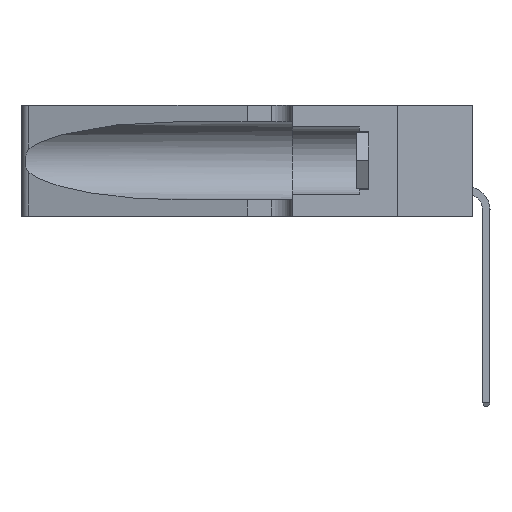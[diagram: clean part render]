
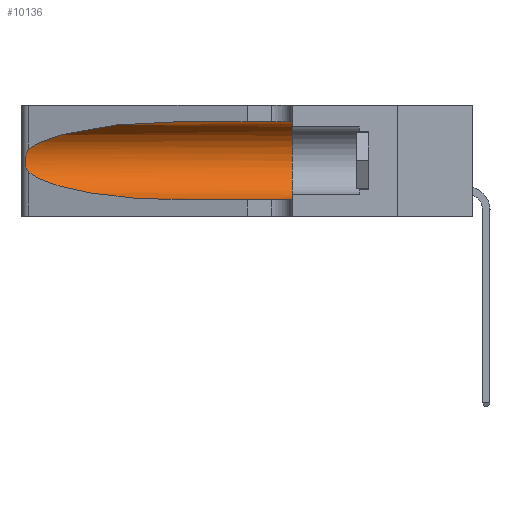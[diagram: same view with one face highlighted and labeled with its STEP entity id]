
A CAD part, left-side view. The second image highlights one B-rep face of the part: STEP entity #10136.
In plain terms, the highlighted cylindrical face has radius 3.308 mm (diameter 6.617 mm), a partial arc.
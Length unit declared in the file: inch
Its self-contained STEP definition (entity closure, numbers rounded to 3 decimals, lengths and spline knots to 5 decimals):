
#160 = AXIS2_PLACEMENT_3D ( 'NONE', #9723, #9544, #17660 ) ;
#424 = CARTESIAN_POINT ( 'NONE',  ( 0.25487, 1.22718, 0.22369 ) ) ;
#760 = CARTESIAN_POINT ( 'NONE',  ( 0.25487, 1.22718, 0.14631 ) ) ;
#923 = VECTOR ( 'NONE', #3979, 39.37008 ) ;
#3380 = EDGE_CURVE ( 'NONE', #23923, #12588, #18305, .T. ) ;
#3622 = CARTESIAN_POINT ( 'NONE',  ( 0.2373, 1.15595, 0.08982 ) ) ;
#3849 = CARTESIAN_POINT ( 'NONE',  ( 0.25639, 1.23186, 0.15144 ) ) ;
#3979 = DIRECTION ( 'NONE',  ( 0., -1., 0. ) ) ;
#3989 = LINE ( 'NONE', #20036, #8132 ) ;
#4037 = EDGE_LOOP ( 'NONE', ( #21198, #19770, #12137, #24321, #8334, #25973 ) ) ;
#4907 =( BOUNDED_CURVE ( )  B_SPLINE_CURVE ( 3, ( #18296, #20183, #20349, #8144 ),
 .UNSPECIFIED., .F., .T. ) 
 B_SPLINE_CURVE_WITH_KNOTS ( ( 4, 4 ),
 ( 1.5708, 2.84003 ),
 .UNSPECIFIED. ) 
 CURVE ( )  GEOMETRIC_REPRESENTATION_ITEM ( )  RATIONAL_B_SPLINE_CURVE ( ( 1., 0.87, 0.87, 1. ) ) 
 REPRESENTATION_ITEM ( '' )  );
#4914 = VERTEX_POINT ( 'NONE', #22704 ) ;
#5888 = CARTESIAN_POINT ( 'NONE',  ( 0.25487, 1.22718, 0.14631 ) ) ;
#6140 = CARTESIAN_POINT ( 'NONE',  ( 0.26075, 1.23896, 0.19203 ) ) ;
#6483 = VERTEX_POINT ( 'NONE', #17457 ) ;
#6554 = CARTESIAN_POINT ( 'NONE',  ( 0.1305, 0.35, 0.185 ) ) ;
#6601 = EDGE_CURVE ( 'NONE', #6483, #23923, #4907, .T. ) ;
#6860 = VERTEX_POINT ( 'NONE', #12199 ) ;
#7233 = CIRCLE ( 'NONE', #8900, 0.13025 ) ;
#8132 = VECTOR ( 'NONE', #14002, 39.37008 ) ;
#8144 = CARTESIAN_POINT ( 'NONE',  ( 0.25487, 1.22718, 0.22369 ) ) ;
#8334 = ORIENTED_EDGE ( 'NONE', *, *, #20590, .F. ) ;
#8588 = CARTESIAN_POINT ( 'NONE',  ( 0.25639, 1.23184, 0.21858 ) ) ;
#8821 =( BOUNDED_CURVE ( )  B_SPLINE_CURVE ( 3, ( #760, #3622, #20801, #24889 ),
 .UNSPECIFIED., .F., .F. ) 
 B_SPLINE_CURVE_WITH_KNOTS ( ( 4, 4 ),
 ( 3.44316, 4.71239 ),
 .UNSPECIFIED. ) 
 CURVE ( )  GEOMETRIC_REPRESENTATION_ITEM ( )  RATIONAL_B_SPLINE_CURVE ( ( 1., 0.87, 0.87, 1. ) ) 
 REPRESENTATION_ITEM ( '' )  );
#8900 = AXIS2_PLACEMENT_3D ( 'NONE', #6554, #14519, #14708 ) ;
#9544 = DIRECTION ( 'NONE',  ( 0., -1., 0. ) ) ;
#9723 = CARTESIAN_POINT ( 'NONE',  ( 0.1305, 1.61858, 0.185 ) ) ;
#9983 = EDGE_CURVE ( 'NONE', #12588, #4914, #8821, .T. ) ;
#10136 = ADVANCED_FACE ( 'NONE', ( #15516 ), #26004, .F. ) ;
#10269 = CARTESIAN_POINT ( 'NONE',  ( 0.25789, 1.23486, 0.15765 ) ) ;
#12137 = ORIENTED_EDGE ( 'NONE', *, *, #9983, .T. ) ;
#12199 = CARTESIAN_POINT ( 'NONE',  ( 0.1305, 0.35, 0.05475 ) ) ;
#12588 = VERTEX_POINT ( 'NONE', #23212 ) ;
#13683 = VERTEX_POINT ( 'NONE', #13829 ) ;
#13829 = CARTESIAN_POINT ( 'NONE',  ( 0.1305, 0.35, 0.31525 ) ) ;
#14002 = DIRECTION ( 'NONE',  ( 0., -1., 0. ) ) ;
#14123 = CARTESIAN_POINT ( 'NONE',  ( 0.25487, 1.22718, 0.22369 ) ) ;
#14519 = DIRECTION ( 'NONE',  ( 0., 1., 0. ) ) ;
#14708 = DIRECTION ( 'NONE',  ( 0., 0., 1. ) ) ;
#15105 = EDGE_CURVE ( 'NONE', #6483, #13683, #21674, .T. ) ;
#15516 = FACE_OUTER_BOUND ( 'NONE', #4037, .T. ) ;
#17457 = CARTESIAN_POINT ( 'NONE',  ( 0.1305, 0.72297, 0.31525 ) ) ;
#17660 = DIRECTION ( 'NONE',  ( 0., 0., -1. ) ) ;
#18105 = CARTESIAN_POINT ( 'NONE',  ( 0.25555, 1.22993, 0.14849 ) ) ;
#18271 = CARTESIAN_POINT ( 'NONE',  ( 0.26018, 1.23835, 0.19895 ) ) ;
#18296 = CARTESIAN_POINT ( 'NONE',  ( 0.1305, 0.72297, 0.31525 ) ) ;
#18305 = B_SPLINE_CURVE_WITH_KNOTS ( 'NONE', 3,
 ( #424, #18836, #8588, #20237, #18362, #18271, #6140, #20414, #22449, #24563, #10269, #3849, #18105, #5888 ),
 .UNSPECIFIED., .F., .F.,
 ( 4, 2, 2, 2, 2, 2, 4 ),
 ( 0., 0.00027, 0.00053, 0.00107, 0.0016, 0.00187, 0.00214 ),
 .UNSPECIFIED. ) ;
#18320 = CARTESIAN_POINT ( 'NONE',  ( 0.1305, 1.61858, 0.31525 ) ) ;
#18362 = CARTESIAN_POINT ( 'NONE',  ( 0.25854, 1.2359, 0.20912 ) ) ;
#18836 = CARTESIAN_POINT ( 'NONE',  ( 0.25555, 1.22994, 0.2215 ) ) ;
#19770 = ORIENTED_EDGE ( 'NONE', *, *, #3380, .T. ) ;
#20036 = CARTESIAN_POINT ( 'NONE',  ( 0.1305, 1.61858, 0.05475 ) ) ;
#20183 = CARTESIAN_POINT ( 'NONE',  ( 0.18966, 0.96281, 0.31525 ) ) ;
#20237 = CARTESIAN_POINT ( 'NONE',  ( 0.25787, 1.23484, 0.2124 ) ) ;
#20349 = CARTESIAN_POINT ( 'NONE',  ( 0.2373, 1.15595, 0.28018 ) ) ;
#20414 = CARTESIAN_POINT ( 'NONE',  ( 0.26075, 1.23896, 0.178 ) ) ;
#20590 = EDGE_CURVE ( 'NONE', #13683, #6860, #7233, .T. ) ;
#20801 = CARTESIAN_POINT ( 'NONE',  ( 0.18966, 0.96281, 0.05475 ) ) ;
#21198 = ORIENTED_EDGE ( 'NONE', *, *, #6601, .T. ) ;
#21674 = LINE ( 'NONE', #18320, #923 ) ;
#22449 = CARTESIAN_POINT ( 'NONE',  ( 0.26017, 1.23833, 0.17102 ) ) ;
#22694 = EDGE_CURVE ( 'NONE', #4914, #6860, #3989, .T. ) ;
#22704 = CARTESIAN_POINT ( 'NONE',  ( 0.1305, 0.72297, 0.05475 ) ) ;
#23212 = CARTESIAN_POINT ( 'NONE',  ( 0.25487, 1.22718, 0.14631 ) ) ;
#23923 = VERTEX_POINT ( 'NONE', #14123 ) ;
#24321 = ORIENTED_EDGE ( 'NONE', *, *, #22694, .T. ) ;
#24563 = CARTESIAN_POINT ( 'NONE',  ( 0.25856, 1.23593, 0.16098 ) ) ;
#24889 = CARTESIAN_POINT ( 'NONE',  ( 0.1305, 0.72297, 0.05475 ) ) ;
#25973 = ORIENTED_EDGE ( 'NONE', *, *, #15105, .F. ) ;
#26004 = CYLINDRICAL_SURFACE ( 'NONE', #160, 0.13025 ) ;
